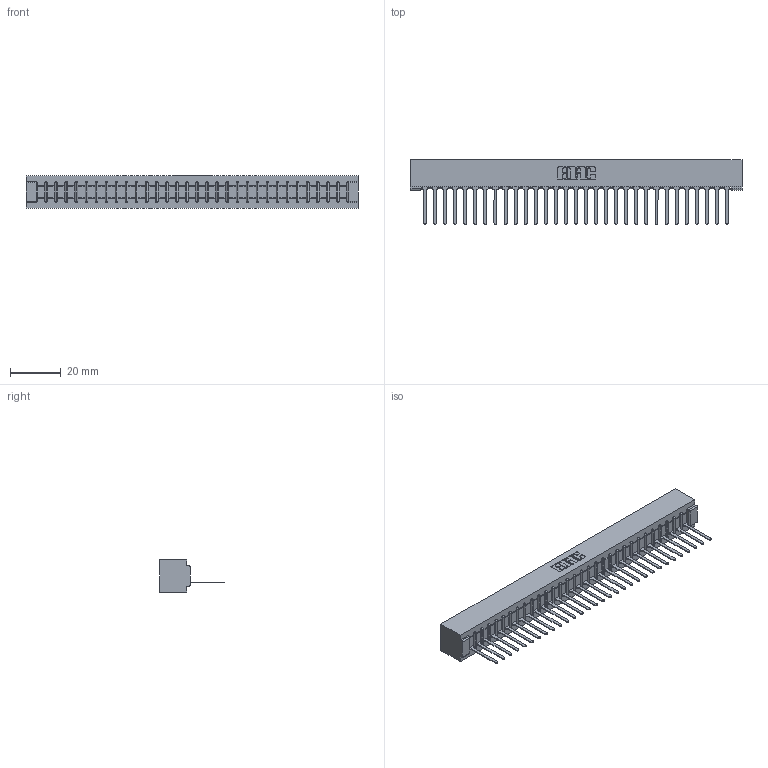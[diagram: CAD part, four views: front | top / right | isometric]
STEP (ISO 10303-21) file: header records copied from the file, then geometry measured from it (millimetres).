
FILE_DESCRIPTION (( 'STEP AP203' ), '1' );
FILE_NAME ('357-031-547-101.STEP', '2019-09-14T04:50:09', ( '' ), ( '' ), 'SwSTEP 2.0', 'SolidWorks 2016', '' );
FILE_SCHEMA (( 'CONFIG_CONTROL_DESIGN' ));
Length unit declared in the file: inch
Products named in the file (3): 357-031-547-101; 307-290-001_547; 307 Part_No Mounting Lugs
Assembly tree (32 placements, depth 2):
  357-031-547-101
    307 Part_No Mounting Lugs
    307-290-001_547  x31
Bounding box: 130.71 x 25.43 x 12.7 mm (x, y, z)
Volume: 14087.3 mm3; surface area: 15380 mm2
Topology: 32 solids, 32 shells, 1878 faces, 5321 edges, 3418 vertices
Faces by surface type: plane 1213, cylinder 601, sphere 64
Entity records: 27622 total; most frequent: CARTESIAN_POINT 4648, ORIENTED_EDGE 4634, DIRECTION 4525, EDGE_CURVE 2317, LINE 1775, VECTOR 1775, VERTEX_POINT 1498, AXIS2_PLACEMENT_3D 1375
